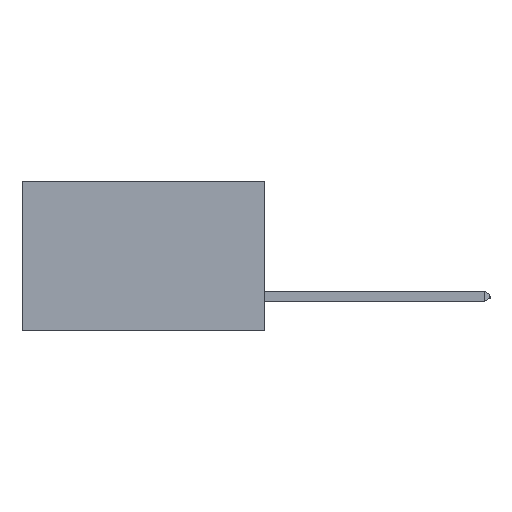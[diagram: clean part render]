
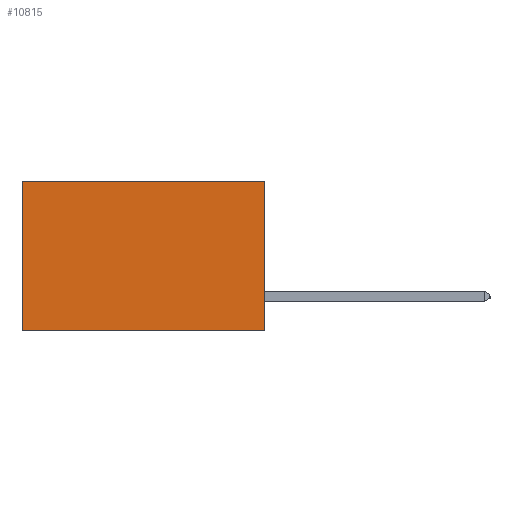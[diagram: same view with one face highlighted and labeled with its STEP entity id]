
A CAD part, left-side view. The second image highlights one B-rep face of the part: STEP entity #10815.
In plain terms, the highlighted planar face has unit normal (-1, 0, 0).
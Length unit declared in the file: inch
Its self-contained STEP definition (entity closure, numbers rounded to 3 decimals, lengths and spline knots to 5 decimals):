
#609 = DIRECTION ( 'NONE',  ( 0., 0., -1. ) ) ;
#747 = VECTOR ( 'NONE', #9300, 39.37008 ) ;
#825 = LINE ( 'NONE', #4451, #5875 ) ;
#985 = ORIENTED_EDGE ( 'NONE', *, *, #3271, .F. ) ;
#1212 = DIRECTION ( 'NONE',  ( 0., 0., -1. ) ) ;
#1804 = LINE ( 'NONE', #13415, #2453 ) ;
#2243 = VERTEX_POINT ( 'NONE', #11020 ) ;
#2453 = VECTOR ( 'NONE', #12616, 39.37008 ) ;
#3071 = CARTESIAN_POINT ( 'NONE',  ( 0.298, 0., -0.37 ) ) ;
#3271 = EDGE_CURVE ( 'NONE', #2243, #11025, #11346, .T. ) ;
#3536 = ORIENTED_EDGE ( 'NONE', *, *, #6222, .F. ) ;
#4451 = CARTESIAN_POINT ( 'NONE',  ( 0.298, 0.6, 0. ) ) ;
#5875 = VECTOR ( 'NONE', #1212, 39.37008 ) ;
#5891 = EDGE_LOOP ( 'NONE', ( #9699, #3536, #985, #7742 ) ) ;
#6222 = EDGE_CURVE ( 'NONE', #11025, #9885, #1804, .T. ) ;
#6704 = FACE_OUTER_BOUND ( 'NONE', #5891, .T. ) ;
#7074 = DIRECTION ( 'NONE',  ( 1., 0., 0. ) ) ;
#7587 = EDGE_CURVE ( 'NONE', #2243, #12163, #8957, .T. ) ;
#7742 = ORIENTED_EDGE ( 'NONE', *, *, #7587, .T. ) ;
#8624 = CARTESIAN_POINT ( 'NONE',  ( 0.298, 0., 0. ) ) ;
#8957 = LINE ( 'NONE', #8624, #747 ) ;
#9144 = CARTESIAN_POINT ( 'NONE',  ( 0.298, 0., 0. ) ) ;
#9300 = DIRECTION ( 'NONE',  ( 0., 1., 0. ) ) ;
#9699 = ORIENTED_EDGE ( 'NONE', *, *, #12563, .T. ) ;
#9820 = AXIS2_PLACEMENT_3D ( 'NONE', #9144, #7074, #609 ) ;
#9885 = VERTEX_POINT ( 'NONE', #13779 ) ;
#10200 = CARTESIAN_POINT ( 'NONE',  ( 0.298, 0.6, 0. ) ) ;
#10683 = VECTOR ( 'NONE', #11589, 39.37008 ) ;
#10815 = ADVANCED_FACE ( 'NONE', ( #6704 ), #13354, .F. ) ;
#11020 = CARTESIAN_POINT ( 'NONE',  ( 0.298, 0., 0. ) ) ;
#11025 = VERTEX_POINT ( 'NONE', #3071 ) ;
#11346 = LINE ( 'NONE', #12733, #10683 ) ;
#11589 = DIRECTION ( 'NONE',  ( 0., 0., -1. ) ) ;
#12163 = VERTEX_POINT ( 'NONE', #10200 ) ;
#12563 = EDGE_CURVE ( 'NONE', #12163, #9885, #825, .T. ) ;
#12616 = DIRECTION ( 'NONE',  ( 0., 1., 0. ) ) ;
#12733 = CARTESIAN_POINT ( 'NONE',  ( 0.298, 0., 0. ) ) ;
#13354 = PLANE ( 'NONE',  #9820 ) ;
#13415 = CARTESIAN_POINT ( 'NONE',  ( 0.298, 0., -0.37 ) ) ;
#13779 = CARTESIAN_POINT ( 'NONE',  ( 0.298, 0.6, -0.37 ) ) ;
